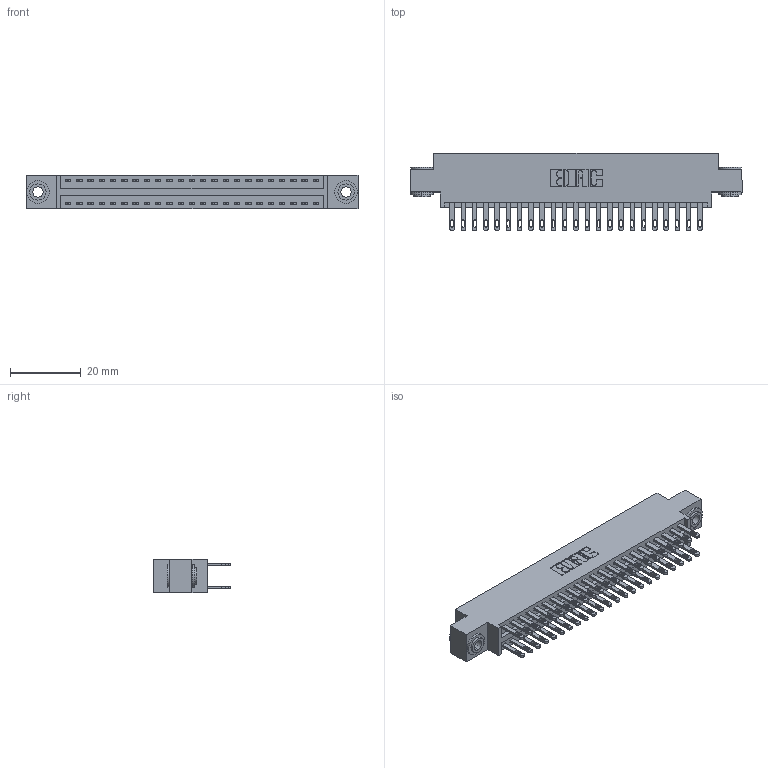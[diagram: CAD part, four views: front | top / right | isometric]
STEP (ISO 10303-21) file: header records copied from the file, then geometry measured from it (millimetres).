
FILE_DESCRIPTION (( 'STEP AP203' ), '1' );
FILE_NAME ('346-046-500-803.STEP', '2018-08-25T04:34:00', ( '' ), ( '' ), 'SwSTEP 2.0', 'SolidWorks 2016', '' );
FILE_SCHEMA (( 'CONFIG_CONTROL_DESIGN' ));
Length unit declared in the file: inch
Products named in the file (4): 346 Part_0.170 Offset - 0.156 Dia-TH; 345-292-001_345-293-100; 345-250-002_345-250-002-102; 346-046-500-803
Assembly tree (49 placements, depth 2):
  346-046-500-803
    346 Part_0.170 Offset - 0.156 Dia-TH
    345-292-001_345-293-100  x46
    345-250-002_345-250-002-102  x2
Bounding box: 93.6 x 21.84 x 9.4 mm (x, y, z)
Volume: 8984.8 mm3; surface area: 12926.9 mm2
Topology: 49 solids, 49 shells, 2372 faces, 7179 edges, 4782 vertices
Faces by surface type: plane 1424, cylinder 940, cone 8
Entity records: 18280 total; most frequent: CARTESIAN_POINT 3015, ORIENTED_EDGE 2942, DIRECTION 2741, EDGE_CURVE 1471, VECTOR 1219, LINE 1219, VERTEX_POINT 978, AXIS2_PLACEMENT_3D 761
